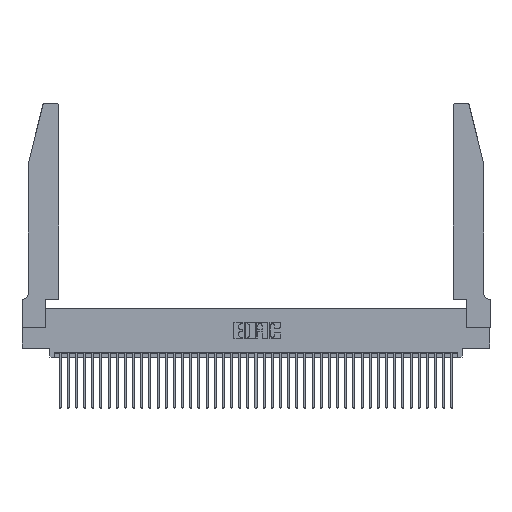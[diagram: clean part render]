
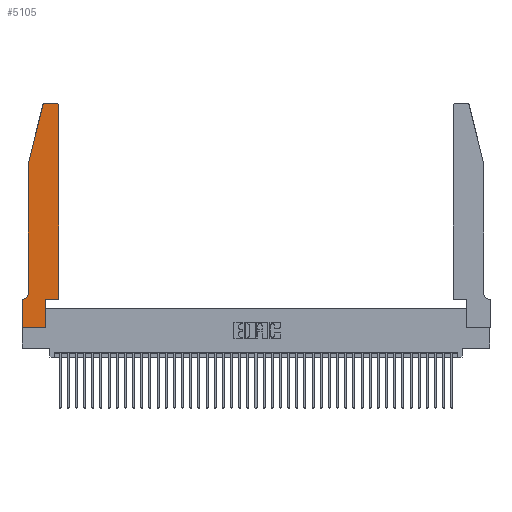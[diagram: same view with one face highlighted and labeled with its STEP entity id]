
A CAD part, top view. The second image highlights one B-rep face of the part: STEP entity #5105.
In plain terms, the highlighted planar face has unit normal (0, 0, 1).
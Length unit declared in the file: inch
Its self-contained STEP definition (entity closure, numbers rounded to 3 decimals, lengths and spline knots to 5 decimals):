
#465 = ORIENTED_EDGE ( 'NONE', *, *, #41729, .T. ) ;
#1363 = VECTOR ( 'NONE', #6825, 39.37008 ) ;
#1501 = EDGE_CURVE ( 'NONE', #1859, #33957, #31683, .T. ) ;
#1859 = VERTEX_POINT ( 'NONE', #15496 ) ;
#2001 = DIRECTION ( 'NONE',  ( 1., 0., 0. ) ) ;
#2087 = CIRCLE ( 'NONE', #3462, 0.07 ) ;
#2096 = EDGE_LOOP ( 'NONE', ( #25030, #6389, #13475, #465, #26836, #38485, #40272, #29037, #37730, #38194, #23747, #35781 ) ) ;
#2851 = CARTESIAN_POINT ( 'NONE',  ( 0.4505, 2.72, 0.37 ) ) ;
#3462 = AXIS2_PLACEMENT_3D ( 'NONE', #9162, #32059, #12432 ) ;
#3631 = LINE ( 'NONE', #24466, #37454 ) ;
#3854 = EDGE_CURVE ( 'NONE', #38340, #14223, #26866, .T. ) ;
#5105 = ADVANCED_FACE ( 'NONE', ( #33962 ), #22141, .T. ) ;
#5238 = CARTESIAN_POINT ( 'NONE',  ( 0.4205, 2.75, 0.37 ) ) ;
#5854 = CARTESIAN_POINT ( 'NONE',  ( 0., 0.35, 0.37 ) ) ;
#6064 = VECTOR ( 'NONE', #18457, 39.37008 ) ;
#6389 = ORIENTED_EDGE ( 'NONE', *, *, #3854, .T. ) ;
#6825 = DIRECTION ( 'NONE',  ( -1., 0., 0. ) ) ;
#7086 = LINE ( 'NONE', #31524, #6064 ) ;
#7852 = EDGE_CURVE ( 'NONE', #41621, #18464, #17876, .T. ) ;
#7924 = EDGE_CURVE ( 'NONE', #18464, #38340, #40954, .T. ) ;
#8197 = DIRECTION ( 'NONE',  ( 1., 0., 0. ) ) ;
#8471 = VECTOR ( 'NONE', #37296, 39.37008 ) ;
#9019 = CARTESIAN_POINT ( 'NONE',  ( 0.0755, 0.42, 0.37 ) ) ;
#9132 = DIRECTION ( 'NONE',  ( 1., 0., 0. ) ) ;
#9162 = CARTESIAN_POINT ( 'NONE',  ( 0.0055, 0.42, 0.37 ) ) ;
#12432 = DIRECTION ( 'NONE',  ( -1., 0., 0. ) ) ;
#12908 = CARTESIAN_POINT ( 'NONE',  ( 0.0055, 0.35, 0.37 ) ) ;
#12998 = VERTEX_POINT ( 'NONE', #17062 ) ;
#13136 = CARTESIAN_POINT ( 'NONE',  ( 0.0755, 2., 0.37 ) ) ;
#13290 = EDGE_CURVE ( 'NONE', #12998, #29066, #25835, .T. ) ;
#13380 = CARTESIAN_POINT ( 'NONE',  ( 0.0755, 0.35, 0.37 ) ) ;
#13475 = ORIENTED_EDGE ( 'NONE', *, *, #19003, .T. ) ;
#14183 = CARTESIAN_POINT ( 'NONE',  ( 0.4205, 2.72, 0.37 ) ) ;
#14223 = VERTEX_POINT ( 'NONE', #18704 ) ;
#14241 = AXIS2_PLACEMENT_3D ( 'NONE', #5854, #28726, #9132 ) ;
#14272 = VECTOR ( 'NONE', #25521, 39.37008 ) ;
#14831 = VECTOR ( 'NONE', #15051, 39.37008 ) ;
#15051 = DIRECTION ( 'NONE',  ( -1., 0., 0. ) ) ;
#15496 = CARTESIAN_POINT ( 'NONE',  ( 0., 0.35, 0.37 ) ) ;
#17062 = CARTESIAN_POINT ( 'NONE',  ( 0.2865, 0., 0.37 ) ) ;
#17436 = DIRECTION ( 'NONE',  ( 1., 0., 0. ) ) ;
#17485 = EDGE_CURVE ( 'NONE', #29066, #24995, #3631, .T. ) ;
#17876 = CIRCLE ( 'NONE', #40197, 0.03 ) ;
#18441 = CARTESIAN_POINT ( 'NONE',  ( 0., 0., 0.37 ) ) ;
#18457 = DIRECTION ( 'NONE',  ( -0.239, -0.971, 0. ) ) ;
#18464 = VERTEX_POINT ( 'NONE', #5238 ) ;
#18704 = CARTESIAN_POINT ( 'NONE',  ( 0.25487, 2.72718, 0.37 ) ) ;
#18706 = VERTEX_POINT ( 'NONE', #12908 ) ;
#19003 = EDGE_CURVE ( 'NONE', #14223, #36199, #7086, .T. ) ;
#19071 = CARTESIAN_POINT ( 'NONE',  ( 0.284, 2.72, 0.37 ) ) ;
#21039 = LINE ( 'NONE', #13136, #38474 ) ;
#21487 = CARTESIAN_POINT ( 'NONE',  ( 0.4505, 0.35, 0.37 ) ) ;
#22141 = PLANE ( 'NONE',  #14241 ) ;
#22371 = DIRECTION ( 'NONE',  ( 1., 0., 0. ) ) ;
#22866 = DIRECTION ( 'NONE',  ( 0., -1., 0. ) ) ;
#23094 = LINE ( 'NONE', #33802, #39536 ) ;
#23612 = VECTOR ( 'NONE', #2001, 39.37008 ) ;
#23747 = ORIENTED_EDGE ( 'NONE', *, *, #41273, .T. ) ;
#24466 = CARTESIAN_POINT ( 'NONE',  ( 0.4505, 0.35, 0.37 ) ) ;
#24639 = LINE ( 'NONE', #18441, #23612 ) ;
#24995 = VERTEX_POINT ( 'NONE', #21487 ) ;
#25030 = ORIENTED_EDGE ( 'NONE', *, *, #7924, .T. ) ;
#25521 = DIRECTION ( 'NONE',  ( 0., -1., 0. ) ) ;
#25835 = LINE ( 'NONE', #33991, #8471 ) ;
#26438 = CARTESIAN_POINT ( 'NONE',  ( 0., 0., 0.37 ) ) ;
#26836 = ORIENTED_EDGE ( 'NONE', *, *, #41580, .T. ) ;
#26866 = CIRCLE ( 'NONE', #35077, 0.03 ) ;
#28726 = DIRECTION ( 'NONE',  ( 0., 0., 1. ) ) ;
#29037 = ORIENTED_EDGE ( 'NONE', *, *, #33634, .T. ) ;
#29066 = VERTEX_POINT ( 'NONE', #36982 ) ;
#31524 = CARTESIAN_POINT ( 'NONE',  ( 0.0755, 2., 0.37 ) ) ;
#31683 = LINE ( 'NONE', #32007, #14272 ) ;
#32007 = CARTESIAN_POINT ( 'NONE',  ( 0., 0., 0.37 ) ) ;
#32059 = DIRECTION ( 'NONE',  ( 0., 0., -1. ) ) ;
#33634 = EDGE_CURVE ( 'NONE', #33957, #12998, #24639, .T. ) ;
#33802 = CARTESIAN_POINT ( 'NONE',  ( 0.4505, 0.35, 0.37 ) ) ;
#33945 = CARTESIAN_POINT ( 'NONE',  ( 0.2605, 2.75, 0.37 ) ) ;
#33957 = VERTEX_POINT ( 'NONE', #26438 ) ;
#33962 = FACE_OUTER_BOUND ( 'NONE', #2096, .T. ) ;
#33991 = CARTESIAN_POINT ( 'NONE',  ( 0.2865, 0.35, 0.37 ) ) ;
#34168 = LINE ( 'NONE', #13380, #1363 ) ;
#34266 = CARTESIAN_POINT ( 'NONE',  ( 0.0755, 2., 0.37 ) ) ;
#35077 = AXIS2_PLACEMENT_3D ( 'NONE', #19071, #42000, #22371 ) ;
#35781 = ORIENTED_EDGE ( 'NONE', *, *, #7852, .T. ) ;
#36199 = VERTEX_POINT ( 'NONE', #34266 ) ;
#36298 = EDGE_CURVE ( 'NONE', #18706, #1859, #34168, .T. ) ;
#36982 = CARTESIAN_POINT ( 'NONE',  ( 0.2865, 0.35, 0.37 ) ) ;
#37112 = DIRECTION ( 'NONE',  ( 0., 0., 1. ) ) ;
#37117 = DIRECTION ( 'NONE',  ( 0., 1., 0. ) ) ;
#37296 = DIRECTION ( 'NONE',  ( 0., 1., 0. ) ) ;
#37454 = VECTOR ( 'NONE', #8197, 39.37008 ) ;
#37730 = ORIENTED_EDGE ( 'NONE', *, *, #13290, .T. ) ;
#38194 = ORIENTED_EDGE ( 'NONE', *, *, #17485, .T. ) ;
#38340 = VERTEX_POINT ( 'NONE', #39820 ) ;
#38474 = VECTOR ( 'NONE', #22866, 39.37008 ) ;
#38485 = ORIENTED_EDGE ( 'NONE', *, *, #36298, .T. ) ;
#39536 = VECTOR ( 'NONE', #37117, 39.37008 ) ;
#39820 = CARTESIAN_POINT ( 'NONE',  ( 0.284, 2.75, 0.37 ) ) ;
#40197 = AXIS2_PLACEMENT_3D ( 'NONE', #14183, #37112, #17436 ) ;
#40272 = ORIENTED_EDGE ( 'NONE', *, *, #1501, .T. ) ;
#40954 = LINE ( 'NONE', #33945, #14831 ) ;
#41273 = EDGE_CURVE ( 'NONE', #24995, #41621, #23094, .T. ) ;
#41543 = VERTEX_POINT ( 'NONE', #9019 ) ;
#41580 = EDGE_CURVE ( 'NONE', #41543, #18706, #2087, .T. ) ;
#41621 = VERTEX_POINT ( 'NONE', #2851 ) ;
#41729 = EDGE_CURVE ( 'NONE', #36199, #41543, #21039, .T. ) ;
#42000 = DIRECTION ( 'NONE',  ( 0., 0., 1. ) ) ;
